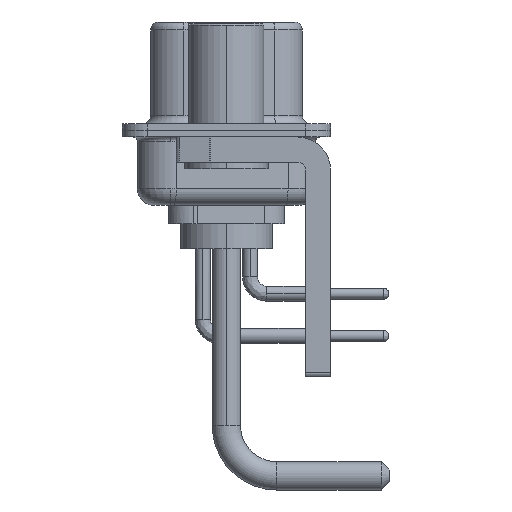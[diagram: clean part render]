
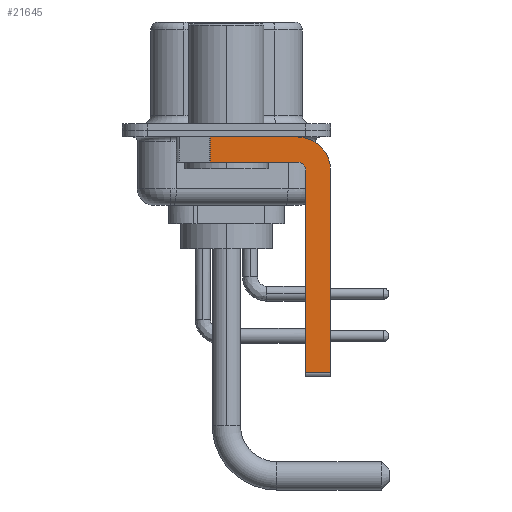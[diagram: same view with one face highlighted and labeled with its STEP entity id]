
A CAD part, left-side view. The second image highlights one B-rep face of the part: STEP entity #21645.
In plain terms, the highlighted planar face has unit normal (-1, 0, 0).
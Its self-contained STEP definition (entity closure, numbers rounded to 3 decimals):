
#722 = VERTEX_POINT ( 'NONE', #23640 ) ;
#1116 = EDGE_CURVE ( 'NONE', #16060, #3705, #30953, .T. ) ;
#1211 = DIRECTION ( 'NONE',  ( 0., 0., 1. ) ) ;
#1762 = DIRECTION ( 'NONE',  ( 0., 0., -1. ) ) ;
#1882 = AXIS2_PLACEMENT_3D ( 'NONE', #25889, #13488, #16460 ) ;
#1963 = EDGE_CURVE ( 'NONE', #16060, #21242, #5042, .T. ) ;
#2169 = LINE ( 'NONE', #21323, #11797 ) ;
#2479 = DIRECTION ( 'NONE',  ( 0., -1., 0. ) ) ;
#3146 = DIRECTION ( 'NONE',  ( 0., -1., 0. ) ) ;
#3540 = LINE ( 'NONE', #17215, #23247 ) ;
#3606 = CARTESIAN_POINT ( 'NONE',  ( -2.9, 0.978, -1.9 ) ) ;
#3705 = VERTEX_POINT ( 'NONE', #26994 ) ;
#4977 = VERTEX_POINT ( 'NONE', #3606 ) ;
#5042 = LINE ( 'NONE', #7552, #13655 ) ;
#5352 = VECTOR ( 'NONE', #1762, 1000. ) ;
#5721 = ORIENTED_EDGE ( 'NONE', *, *, #1116, .F. ) ;
#5896 = VERTEX_POINT ( 'NONE', #9356 ) ;
#6557 = DIRECTION ( 'NONE',  ( -1., 0., 0. ) ) ;
#6780 = CARTESIAN_POINT ( 'NONE',  ( -2.9, 0.978, -1.9 ) ) ;
#6915 = ORIENTED_EDGE ( 'NONE', *, *, #9423, .F. ) ;
#7552 = CARTESIAN_POINT ( 'NONE',  ( -2.9, -4.25, -14.55 ) ) ;
#7776 = LINE ( 'NONE', #13368, #10036 ) ;
#8091 = EDGE_CURVE ( 'NONE', #12814, #4977, #7776, .T. ) ;
#9356 = CARTESIAN_POINT ( 'NONE',  ( -2.9, -6.25, -2.4 ) ) ;
#9423 = EDGE_CURVE ( 'NONE', #5896, #21242, #3540, .T. ) ;
#10036 = VECTOR ( 'NONE', #17210, 1000. ) ;
#11797 = VECTOR ( 'NONE', #2479, 1000. ) ;
#12814 = VERTEX_POINT ( 'NONE', #13265 ) ;
#13265 = CARTESIAN_POINT ( 'NONE',  ( -2.9, -4.25, -1.9 ) ) ;
#13368 = CARTESIAN_POINT ( 'NONE',  ( -2.9, -4.25, -1.9 ) ) ;
#13470 = DIRECTION ( 'NONE',  ( 0., 0., -1. ) ) ;
#13488 = DIRECTION ( 'NONE',  ( 1., 0., 0. ) ) ;
#13655 = VECTOR ( 'NONE', #3146, 1000. ) ;
#13768 = CARTESIAN_POINT ( 'NONE',  ( -2.9, -4.25, -0.4 ) ) ;
#13848 = CARTESIAN_POINT ( 'NONE',  ( -2.9, -4.75, -14.8 ) ) ;
#14428 = ORIENTED_EDGE ( 'NONE', *, *, #8091, .F. ) ;
#14678 = AXIS2_PLACEMENT_3D ( 'NONE', #18337, #6557, #1211 ) ;
#15960 = EDGE_CURVE ( 'NONE', #27694, #5896, #24767, .T. ) ;
#16060 = VERTEX_POINT ( 'NONE', #20710 ) ;
#16460 = DIRECTION ( 'NONE',  ( 0., 0., -1. ) ) ;
#17210 = DIRECTION ( 'NONE',  ( 0., 1., 0. ) ) ;
#17215 = CARTESIAN_POINT ( 'NONE',  ( -2.9, -6.25, -2.4 ) ) ;
#17256 = AXIS2_PLACEMENT_3D ( 'NONE', #18506, #27616, #13470 ) ;
#17439 = EDGE_CURVE ( 'NONE', #722, #27694, #2169, .T. ) ;
#17586 = ORIENTED_EDGE ( 'NONE', *, *, #1963, .T. ) ;
#18310 = ORIENTED_EDGE ( 'NONE', *, *, #15960, .F. ) ;
#18337 = CARTESIAN_POINT ( 'NONE',  ( -2.9, -4.25, -2.4 ) ) ;
#18506 = CARTESIAN_POINT ( 'NONE',  ( -2.9, -4.25, -2.4 ) ) ;
#18675 = ORIENTED_EDGE ( 'NONE', *, *, #27674, .F. ) ;
#18882 = LINE ( 'NONE', #6780, #5352 ) ;
#20022 = DIRECTION ( 'NONE',  ( 0., 0., -1. ) ) ;
#20710 = CARTESIAN_POINT ( 'NONE',  ( -2.9, -4.75, -14.55 ) ) ;
#21242 = VERTEX_POINT ( 'NONE', #21625 ) ;
#21323 = CARTESIAN_POINT ( 'NONE',  ( -2.9, 3., -0.4 ) ) ;
#21625 = CARTESIAN_POINT ( 'NONE',  ( -2.9, -6.25, -14.55 ) ) ;
#21645 = ADVANCED_FACE ( 'NONE', ( #30756 ), #26201, .F. ) ;
#21793 = ORIENTED_EDGE ( 'NONE', *, *, #17439, .F. ) ;
#23247 = VECTOR ( 'NONE', #20022, 1000. ) ;
#23640 = CARTESIAN_POINT ( 'NONE',  ( -2.9, 0.978, -0.4 ) ) ;
#24767 = CIRCLE ( 'NONE', #17256, 2. ) ;
#25098 = ORIENTED_EDGE ( 'NONE', *, *, #28809, .T. ) ;
#25889 = CARTESIAN_POINT ( 'NONE',  ( -2.9, -4.25, -2.4 ) ) ;
#25938 = DIRECTION ( 'NONE',  ( 0., 0., 1. ) ) ;
#26201 = PLANE ( 'NONE',  #1882 ) ;
#26627 = VECTOR ( 'NONE', #25938, 1000. ) ;
#26994 = CARTESIAN_POINT ( 'NONE',  ( -2.9, -4.75, -2.4 ) ) ;
#27616 = DIRECTION ( 'NONE',  ( 1., 0., 0. ) ) ;
#27674 = EDGE_CURVE ( 'NONE', #3705, #12814, #28200, .T. ) ;
#27694 = VERTEX_POINT ( 'NONE', #13768 ) ;
#28200 = CIRCLE ( 'NONE', #14678, 0.5 ) ;
#28809 = EDGE_CURVE ( 'NONE', #722, #4977, #18882, .T. ) ;
#30410 = EDGE_LOOP ( 'NONE', ( #21793, #25098, #14428, #18675, #5721, #17586, #6915, #18310 ) ) ;
#30756 = FACE_OUTER_BOUND ( 'NONE', #30410, .T. ) ;
#30953 = LINE ( 'NONE', #13848, #26627 ) ;
